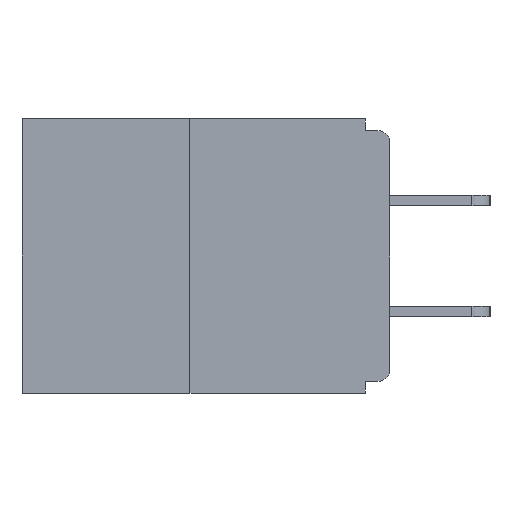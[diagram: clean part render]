
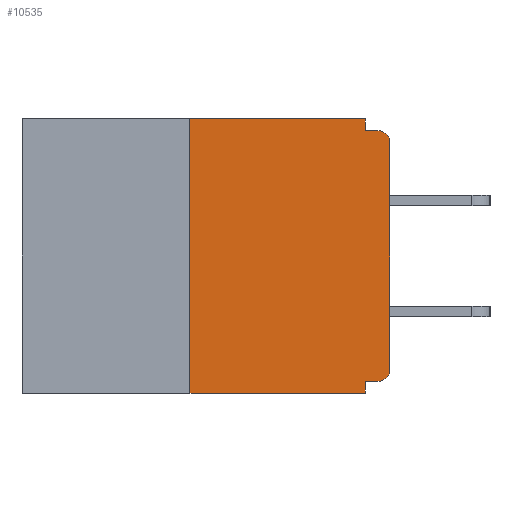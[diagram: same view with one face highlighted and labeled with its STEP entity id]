
A CAD part, left-side view. The second image highlights one B-rep face of the part: STEP entity #10535.
In plain terms, the highlighted planar face has unit normal (-1, 0, 0).
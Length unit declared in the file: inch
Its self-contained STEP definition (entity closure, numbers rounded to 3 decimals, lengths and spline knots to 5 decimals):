
#8 = FACE_OUTER_BOUND ( 'NONE', #28272, .T. ) ;
#28 = CIRCLE ( 'NONE', #18934, 0.015 ) ;
#314 = PLANE ( 'NONE',  #10077 ) ;
#323 = VERTEX_POINT ( 'NONE', #1710 ) ;
#460 = CARTESIAN_POINT ( 'NONE',  ( 0., 0., -0.03 ) ) ;
#1036 = CARTESIAN_POINT ( 'NONE',  ( 0., 0.015, -0.015 ) ) ;
#1472 = DIRECTION ( 'NONE',  ( 0., 0., 1. ) ) ;
#1622 = LINE ( 'NONE', #23385, #2842 ) ;
#1623 = EDGE_CURVE ( 'NONE', #25963, #323, #28, .T. ) ;
#1710 = CARTESIAN_POINT ( 'NONE',  ( 0., 0., -0.313 ) ) ;
#1738 = VECTOR ( 'NONE', #11589, 39.37008 ) ;
#2078 = ORIENTED_EDGE ( 'NONE', *, *, #2791, .F. ) ;
#2365 = VECTOR ( 'NONE', #11010, 39.37008 ) ;
#2791 = EDGE_CURVE ( 'NONE', #26627, #7265, #3073, .T. ) ;
#2842 = VECTOR ( 'NONE', #18933, 39.37008 ) ;
#3073 = LINE ( 'NONE', #12724, #3275 ) ;
#3275 = VECTOR ( 'NONE', #1472, 39.37008 ) ;
#3277 = EDGE_CURVE ( 'NONE', #3788, #9990, #21886, .T. ) ;
#3596 = VECTOR ( 'NONE', #6083, 39.37008 ) ;
#3688 = EDGE_CURVE ( 'NONE', #7265, #3788, #15350, .T. ) ;
#3788 = VERTEX_POINT ( 'NONE', #12893 ) ;
#4166 = DIRECTION ( 'NONE',  ( -1., 0., 0. ) ) ;
#4682 = VECTOR ( 'NONE', #26186, 39.37008 ) ;
#4779 = DIRECTION ( 'NONE',  ( 1., 0., 0. ) ) ;
#5376 = CARTESIAN_POINT ( 'NONE',  ( 0., 0., 0. ) ) ;
#5946 = ORIENTED_EDGE ( 'NONE', *, *, #28276, .T. ) ;
#6083 = DIRECTION ( 'NONE',  ( 0., 1., 0. ) ) ;
#6327 = CARTESIAN_POINT ( 'NONE',  ( 0., 0.031, -0.343 ) ) ;
#6903 = VERTEX_POINT ( 'NONE', #460 ) ;
#7147 = EDGE_CURVE ( 'NONE', #6903, #12540, #23282, .T. ) ;
#7163 = EDGE_CURVE ( 'NONE', #24895, #20366, #11090, .T. ) ;
#7265 = VERTEX_POINT ( 'NONE', #24645 ) ;
#8029 = CARTESIAN_POINT ( 'NONE',  ( 0., 0.031, -0.343 ) ) ;
#8943 = CARTESIAN_POINT ( 'NONE',  ( 0., 0.015, -0.328 ) ) ;
#9763 = ORIENTED_EDGE ( 'NONE', *, *, #7147, .T. ) ;
#9990 = VERTEX_POINT ( 'NONE', #15135 ) ;
#10077 = AXIS2_PLACEMENT_3D ( 'NONE', #15576, #4779, #24240 ) ;
#10535 = ADVANCED_FACE ( 'NONE', ( #8 ), #314, .F. ) ;
#11010 = DIRECTION ( 'NONE',  ( 0., -1., 0. ) ) ;
#11090 = LINE ( 'NONE', #6327, #27417 ) ;
#11522 = CARTESIAN_POINT ( 'NONE',  ( 0., 0.031, -0.328 ) ) ;
#11589 = DIRECTION ( 'NONE',  ( 0., 0., 1. ) ) ;
#11802 = CARTESIAN_POINT ( 'NONE',  ( 0., 0.015, -0.313 ) ) ;
#12310 = ORIENTED_EDGE ( 'NONE', *, *, #17018, .T. ) ;
#12540 = VERTEX_POINT ( 'NONE', #1036 ) ;
#12724 = CARTESIAN_POINT ( 'NONE',  ( 0., 0.25, 0. ) ) ;
#12857 = CARTESIAN_POINT ( 'NONE',  ( 0., 0., -0.015 ) ) ;
#12893 = CARTESIAN_POINT ( 'NONE',  ( 0., 0.031, 0. ) ) ;
#13257 = DIRECTION ( 'NONE',  ( 0., 0., -1. ) ) ;
#14113 = DIRECTION ( 'NONE',  ( 0., 0., -1. ) ) ;
#15072 = ORIENTED_EDGE ( 'NONE', *, *, #7163, .F. ) ;
#15087 = CARTESIAN_POINT ( 'NONE',  ( 0., 0.031, 0. ) ) ;
#15135 = CARTESIAN_POINT ( 'NONE',  ( 0., 0.031, -0.015 ) ) ;
#15350 = LINE ( 'NONE', #26454, #2365 ) ;
#15576 = CARTESIAN_POINT ( 'NONE',  ( 0., 0.46, 0. ) ) ;
#17018 = EDGE_CURVE ( 'NONE', #323, #6903, #25144, .T. ) ;
#17045 = LINE ( 'NONE', #25843, #3596 ) ;
#17200 = EDGE_CURVE ( 'NONE', #25963, #24895, #17045, .T. ) ;
#17622 = DIRECTION ( 'NONE',  ( 0., -1., 0. ) ) ;
#17866 = ORIENTED_EDGE ( 'NONE', *, *, #17200, .F. ) ;
#18933 = DIRECTION ( 'NONE',  ( 0., -1., 0. ) ) ;
#18934 = AXIS2_PLACEMENT_3D ( 'NONE', #11802, #27219, #14113 ) ;
#19437 = EDGE_CURVE ( 'NONE', #9990, #12540, #21658, .T. ) ;
#19754 = DIRECTION ( 'NONE',  ( 0., 0., -1. ) ) ;
#19781 = VECTOR ( 'NONE', #17622, 39.37008 ) ;
#20366 = VERTEX_POINT ( 'NONE', #8029 ) ;
#21658 = LINE ( 'NONE', #12857, #19781 ) ;
#21785 = CARTESIAN_POINT ( 'NONE',  ( 0., 0.015, -0.03 ) ) ;
#21886 = LINE ( 'NONE', #15087, #4682 ) ;
#22592 = CARTESIAN_POINT ( 'NONE',  ( 0., 0.25, -0.343 ) ) ;
#23282 = CIRCLE ( 'NONE', #26966, 0.015 ) ;
#23385 = CARTESIAN_POINT ( 'NONE',  ( 0., 0.46, -0.343 ) ) ;
#24240 = DIRECTION ( 'NONE',  ( 0., 0., -1. ) ) ;
#24645 = CARTESIAN_POINT ( 'NONE',  ( 0., 0.25, 0. ) ) ;
#24660 = ORIENTED_EDGE ( 'NONE', *, *, #19437, .F. ) ;
#24814 = ORIENTED_EDGE ( 'NONE', *, *, #3277, .F. ) ;
#24895 = VERTEX_POINT ( 'NONE', #11522 ) ;
#24935 = ORIENTED_EDGE ( 'NONE', *, *, #1623, .T. ) ;
#25144 = LINE ( 'NONE', #5376, #1738 ) ;
#25843 = CARTESIAN_POINT ( 'NONE',  ( 0., 0., -0.328 ) ) ;
#25963 = VERTEX_POINT ( 'NONE', #8943 ) ;
#26186 = DIRECTION ( 'NONE',  ( 0., 0., -1. ) ) ;
#26454 = CARTESIAN_POINT ( 'NONE',  ( 0., 0.46, 0. ) ) ;
#26559 = ORIENTED_EDGE ( 'NONE', *, *, #3688, .F. ) ;
#26627 = VERTEX_POINT ( 'NONE', #22592 ) ;
#26966 = AXIS2_PLACEMENT_3D ( 'NONE', #21785, #4166, #13257 ) ;
#27219 = DIRECTION ( 'NONE',  ( -1., 0., 0. ) ) ;
#27417 = VECTOR ( 'NONE', #19754, 39.37008 ) ;
#28272 = EDGE_LOOP ( 'NONE', ( #26559, #2078, #5946, #15072, #17866, #24935, #12310, #9763, #24660, #24814 ) ) ;
#28276 = EDGE_CURVE ( 'NONE', #26627, #20366, #1622, .T. ) ;
